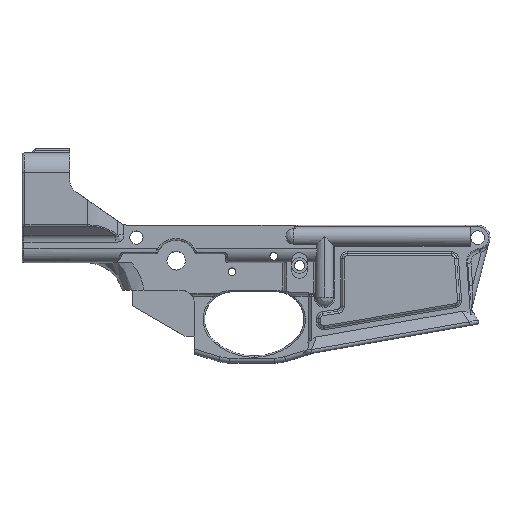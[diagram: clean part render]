
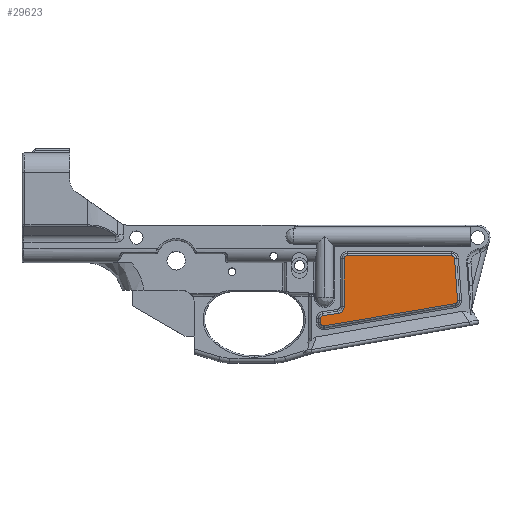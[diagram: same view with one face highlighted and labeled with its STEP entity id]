
A CAD part, top view. The second image highlights one B-rep face of the part: STEP entity #29623.
In plain terms, the highlighted planar face has unit normal (0, 0, 1).
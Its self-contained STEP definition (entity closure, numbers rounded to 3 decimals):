
#1423 = EDGE_CURVE ( 'NONE', #13987, #33959, #15838, .T. ) ;
#1798 = VERTEX_POINT ( 'NONE', #11160 ) ;
#1935 = CARTESIAN_POINT ( 'NONE',  ( 125.626, -42.111, 14.866 ) ) ;
#2079 = EDGE_CURVE ( 'NONE', #41800, #33906, #25573, .T. ) ;
#2340 = EDGE_CURVE ( 'NONE', #19944, #28735, #20647, .T. ) ;
#2350 = DIRECTION ( 'NONE',  ( -1., 0., 0. ) ) ;
#2567 = FACE_OUTER_BOUND ( 'NONE', #32490, .T. ) ;
#2954 = DIRECTION ( 'NONE',  ( 0., -1., 0. ) ) ;
#3045 = DIRECTION ( 'NONE',  ( 0., -1., 0. ) ) ;
#5232 = VECTOR ( 'NONE', #24728, 1000. ) ;
#5422 = DIRECTION ( 'NONE',  ( 0., -1., 0. ) ) ;
#6111 = AXIS2_PLACEMENT_3D ( 'NONE', #1935, #26341, #5422 ) ;
#6360 = EDGE_CURVE ( 'NONE', #28735, #23918, #26058, .T. ) ;
#6689 = CIRCLE ( 'NONE', #26779, 1.524 ) ;
#7025 = VERTEX_POINT ( 'NONE', #24478 ) ;
#7204 = CIRCLE ( 'NONE', #27188, 1.524 ) ;
#7854 = CARTESIAN_POINT ( 'NONE',  ( 125.881, -43.613, 14.866 ) ) ;
#7938 = CARTESIAN_POINT ( 'NONE',  ( 56.966, -53.496, 14.866 ) ) ;
#8383 = EDGE_CURVE ( 'NONE', #23918, #15422, #7204, .T. ) ;
#9216 = CARTESIAN_POINT ( 'NONE',  ( 58.49, -53.496, 14.866 ) ) ;
#10523 = CARTESIAN_POINT ( 'NONE',  ( 124.043, -20.597, 14.866 ) ) ;
#11160 = CARTESIAN_POINT ( 'NONE',  ( 70.583, -19.073, 14.866 ) ) ;
#11342 = CIRCLE ( 'NONE', #23635, 3.556 ) ;
#11778 = DIRECTION ( 'NONE',  ( 0., 0., 1. ) ) ;
#11895 = CARTESIAN_POINT ( 'NONE',  ( 125.562, -20.485, 14.866 ) ) ;
#12654 = VERTEX_POINT ( 'NONE', #21921 ) ;
#12691 = DIRECTION ( 'NONE',  ( 0., -1., 0. ) ) ;
#12809 = CARTESIAN_POINT ( 'NONE',  ( 70.583, -20.597, 14.866 ) ) ;
#13048 = CIRCLE ( 'NONE', #6111, 1.524 ) ;
#13405 = EDGE_CURVE ( 'NONE', #33906, #25845, #42188, .T. ) ;
#13987 = VERTEX_POINT ( 'NONE', #42751 ) ;
#14023 = DIRECTION ( 'NONE',  ( 0., -1., 0. ) ) ;
#14183 = CARTESIAN_POINT ( 'NONE',  ( 124.043, -19.073, 14.866 ) ) ;
#14804 = ORIENTED_EDGE ( 'NONE', *, *, #43253, .T. ) ;
#14928 = EDGE_CURVE ( 'NONE', #33959, #12654, #11342, .T. ) ;
#15422 = VERTEX_POINT ( 'NONE', #42737 ) ;
#15838 = LINE ( 'NONE', #36743, #42536 ) ;
#15888 = DIRECTION ( 'NONE',  ( 0., -1., 0. ) ) ;
#16289 = AXIS2_PLACEMENT_3D ( 'NONE', #32643, #11778, #36123 ) ;
#16321 = DIRECTION ( 'NONE',  ( 0., -1., 0. ) ) ;
#16824 = EDGE_CURVE ( 'NONE', #1798, #13987, #6689, .T. ) ;
#17115 = ORIENTED_EDGE ( 'NONE', *, *, #16824, .T. ) ;
#17389 = CARTESIAN_POINT ( 'NONE',  ( 56.966, -53.496, 14.866 ) ) ;
#17676 = DIRECTION ( 'NONE',  ( 0., 0., 1. ) ) ;
#17787 = ORIENTED_EDGE ( 'NONE', *, *, #14928, .T. ) ;
#18139 = ORIENTED_EDGE ( 'NONE', *, *, #1423, .T. ) ;
#18384 = EDGE_CURVE ( 'NONE', #22675, #19944, #42055, .T. ) ;
#18417 = AXIS2_PLACEMENT_3D ( 'NONE', #44706, #23874, #2954 ) ;
#18645 = CARTESIAN_POINT ( 'NONE',  ( 69.059, -45.099, 14.866 ) ) ;
#19222 = DIRECTION ( 'NONE',  ( -0.073, 0.997, 0. ) ) ;
#19584 = EDGE_CURVE ( 'NONE', #7025, #41800, #13048, .T. ) ;
#19944 = VERTEX_POINT ( 'NONE', #24497 ) ;
#20647 = LINE ( 'NONE', #17389, #39154 ) ;
#21921 = CARTESIAN_POINT ( 'NONE',  ( 66.013, -48.618, 14.866 ) ) ;
#22017 = ORIENTED_EDGE ( 'NONE', *, *, #2340, .T. ) ;
#22675 = VERTEX_POINT ( 'NONE', #41677 ) ;
#22698 = AXIS2_PLACEMENT_3D ( 'NONE', #10523, #34898, #14023 ) ;
#23635 = AXIS2_PLACEMENT_3D ( 'NONE', #44786, #23967, #3045 ) ;
#23874 = DIRECTION ( 'NONE',  ( 0., 0., 1. ) ) ;
#23918 = VERTEX_POINT ( 'NONE', #25468 ) ;
#23967 = DIRECTION ( 'NONE',  ( 0., 0., -1. ) ) ;
#24478 = CARTESIAN_POINT ( 'NONE',  ( 125.881, -43.613, 14.866 ) ) ;
#24497 = CARTESIAN_POINT ( 'NONE',  ( 56.966, -51.249, 14.866 ) ) ;
#24559 = EDGE_CURVE ( 'NONE', #15422, #7025, #29061, .T. ) ;
#24587 = ORIENTED_EDGE ( 'NONE', *, *, #19584, .T. ) ;
#24728 = DIRECTION ( 'NONE',  ( -0.99, -0.144, 0. ) ) ;
#25468 = CARTESIAN_POINT ( 'NONE',  ( 58.49, -55.02, 14.866 ) ) ;
#25573 = LINE ( 'NONE', #29579, #34818 ) ;
#25845 = VERTEX_POINT ( 'NONE', #14183 ) ;
#26058 = CIRCLE ( 'NONE', #16289, 1.524 ) ;
#26341 = DIRECTION ( 'NONE',  ( 0., 0., 1. ) ) ;
#26529 = ORIENTED_EDGE ( 'NONE', *, *, #24559, .T. ) ;
#26779 = AXIS2_PLACEMENT_3D ( 'NONE', #12809, #37175, #16321 ) ;
#27188 = AXIS2_PLACEMENT_3D ( 'NONE', #38519, #17676, #42621 ) ;
#27491 = ORIENTED_EDGE ( 'NONE', *, *, #2079, .T. ) ;
#28735 = VERTEX_POINT ( 'NONE', #7938 ) ;
#29061 = LINE ( 'NONE', #7854, #37192 ) ;
#29579 = CARTESIAN_POINT ( 'NONE',  ( 125.562, -20.485, 14.866 ) ) ;
#29623 = ADVANCED_FACE ( 'NONE', ( #2567 ), #36927, .T. ) ;
#29643 = VECTOR ( 'NONE', #2350, 1000. ) ;
#31731 = AXIS2_PLACEMENT_3D ( 'NONE', #9216, #33592, #12691 ) ;
#32490 = EDGE_LOOP ( 'NONE', ( #35137, #22017, #43274, #36342, #26529, #24587, #27491, #36973, #34125, #17115, #18139, #17787, #14804 ) ) ;
#32643 = CARTESIAN_POINT ( 'NONE',  ( 58.49, -53.496, 14.866 ) ) ;
#33068 = LINE ( 'NONE', #38579, #5232 ) ;
#33592 = DIRECTION ( 'NONE',  ( 0., 0., 1. ) ) ;
#33906 = VERTEX_POINT ( 'NONE', #11895 ) ;
#33959 = VERTEX_POINT ( 'NONE', #18645 ) ;
#34125 = ORIENTED_EDGE ( 'NONE', *, *, #38338, .T. ) ;
#34818 = VECTOR ( 'NONE', #19222, 1000. ) ;
#34898 = DIRECTION ( 'NONE',  ( 0., 0., 1. ) ) ;
#35137 = ORIENTED_EDGE ( 'NONE', *, *, #18384, .T. ) ;
#36123 = DIRECTION ( 'NONE',  ( 0., -1., 0. ) ) ;
#36342 = ORIENTED_EDGE ( 'NONE', *, *, #8383, .T. ) ;
#36743 = CARTESIAN_POINT ( 'NONE',  ( 69.059, -45.099, 14.866 ) ) ;
#36927 = PLANE ( 'NONE',  #31731 ) ;
#36973 = ORIENTED_EDGE ( 'NONE', *, *, #13405, .T. ) ;
#37175 = DIRECTION ( 'NONE',  ( 0., 0., 1. ) ) ;
#37192 = VECTOR ( 'NONE', #42582, 1000. ) ;
#38338 = EDGE_CURVE ( 'NONE', #25845, #1798, #39960, .T. ) ;
#38519 = CARTESIAN_POINT ( 'NONE',  ( 58.49, -53.496, 14.866 ) ) ;
#38579 = CARTESIAN_POINT ( 'NONE',  ( 58.271, -49.741, 14.866 ) ) ;
#39154 = VECTOR ( 'NONE', #41727, 1000. ) ;
#39960 = LINE ( 'NONE', #44108, #29643 ) ;
#41677 = CARTESIAN_POINT ( 'NONE',  ( 58.271, -49.741, 14.866 ) ) ;
#41727 = DIRECTION ( 'NONE',  ( 0., -1., 0. ) ) ;
#41800 = VERTEX_POINT ( 'NONE', #43771 ) ;
#42055 = CIRCLE ( 'NONE', #18417, 1.524 ) ;
#42188 = CIRCLE ( 'NONE', #22698, 1.524 ) ;
#42536 = VECTOR ( 'NONE', #15888, 1000. ) ;
#42582 = DIRECTION ( 'NONE',  ( 0.986, 0.167, 0. ) ) ;
#42621 = DIRECTION ( 'NONE',  ( 0., -1., 0. ) ) ;
#42737 = CARTESIAN_POINT ( 'NONE',  ( 58.744, -54.998, 14.866 ) ) ;
#42751 = CARTESIAN_POINT ( 'NONE',  ( 69.059, -20.597, 14.866 ) ) ;
#43253 = EDGE_CURVE ( 'NONE', #12654, #22675, #33068, .T. ) ;
#43274 = ORIENTED_EDGE ( 'NONE', *, *, #6360, .T. ) ;
#43771 = CARTESIAN_POINT ( 'NONE',  ( 127.146, -41.999, 14.866 ) ) ;
#44108 = CARTESIAN_POINT ( 'NONE',  ( 70.583, -19.073, 14.866 ) ) ;
#44706 = CARTESIAN_POINT ( 'NONE',  ( 58.49, -51.249, 14.866 ) ) ;
#44786 = CARTESIAN_POINT ( 'NONE',  ( 65.503, -45.099, 14.866 ) ) ;
